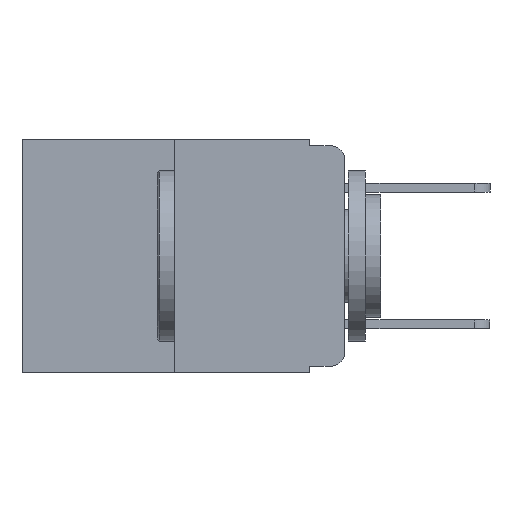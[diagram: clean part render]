
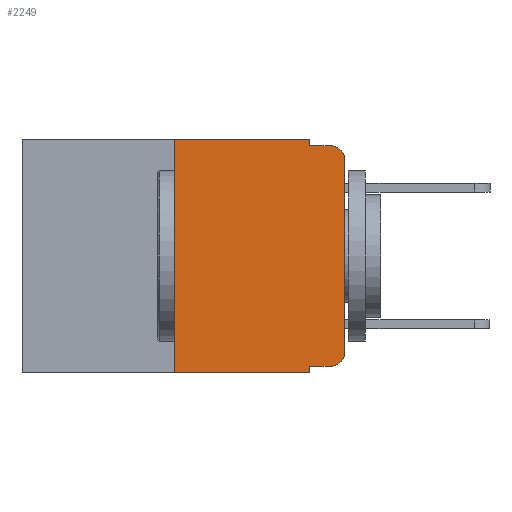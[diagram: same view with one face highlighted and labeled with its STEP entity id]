
A CAD part, left-side view. The second image highlights one B-rep face of the part: STEP entity #2249.
In plain terms, the highlighted planar face has unit normal (-1, 0, 0).
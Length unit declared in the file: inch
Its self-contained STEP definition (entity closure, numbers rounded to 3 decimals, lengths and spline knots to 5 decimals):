
#480 = EDGE_CURVE ( 'NONE', #8708, #18263, #1794, .T. ) ;
#483 = AXIS2_PLACEMENT_3D ( 'NONE', #12032, #5320, #19018 ) ;
#744 = ORIENTED_EDGE ( 'NONE', *, *, #20288, .T. ) ;
#779 = CARTESIAN_POINT ( 'NONE',  ( 0., 0.473, 0. ) ) ;
#816 = ORIENTED_EDGE ( 'NONE', *, *, #19317, .T. ) ;
#1159 = DIRECTION ( 'NONE',  ( 0., -1., 0. ) ) ;
#1303 = ORIENTED_EDGE ( 'NONE', *, *, #17407, .F. ) ;
#1390 = ORIENTED_EDGE ( 'NONE', *, *, #16434, .F. ) ;
#1794 = LINE ( 'NONE', #779, #18004 ) ;
#1799 = ORIENTED_EDGE ( 'NONE', *, *, #480, .F. ) ;
#2011 = LINE ( 'NONE', #6317, #17762 ) ;
#2203 = ORIENTED_EDGE ( 'NONE', *, *, #15414, .F. ) ;
#2249 = ADVANCED_FACE ( 'NONE', ( #18419 ), #9870, .F. ) ;
#2331 = ORIENTED_EDGE ( 'NONE', *, *, #13594, .T. ) ;
#2393 = VERTEX_POINT ( 'NONE', #16743 ) ;
#2771 = DIRECTION ( 'NONE',  ( 0., 0., -1. ) ) ;
#3167 = ORIENTED_EDGE ( 'NONE', *, *, #13340, .F. ) ;
#3249 = CARTESIAN_POINT ( 'NONE',  ( 0., 0.25, 0. ) ) ;
#3755 = ORIENTED_EDGE ( 'NONE', *, *, #12309, .T. ) ;
#3802 = CARTESIAN_POINT ( 'NONE',  ( 0., 0., 0. ) ) ;
#4466 = CARTESIAN_POINT ( 'NONE',  ( 0., 0.051, 0. ) ) ;
#4470 = ORIENTED_EDGE ( 'NONE', *, *, #10319, .T. ) ;
#5081 = VERTEX_POINT ( 'NONE', #13140 ) ;
#5320 = DIRECTION ( 'NONE',  ( 1., 0., 0. ) ) ;
#5491 = DIRECTION ( 'NONE',  ( 0., -1., 0. ) ) ;
#6166 = VECTOR ( 'NONE', #10383, 39.37008 ) ;
#6317 = CARTESIAN_POINT ( 'NONE',  ( 0., 0.051, 0. ) ) ;
#7410 = DIRECTION ( 'NONE',  ( -1., 0., 0. ) ) ;
#7640 = CARTESIAN_POINT ( 'NONE',  ( 0., 0.02, -0.333 ) ) ;
#7674 = EDGE_LOOP ( 'NONE', ( #744, #816, #1303, #1390, #1799, #2203, #2331, #3167, #3755, #4470 ) ) ;
#8078 = LINE ( 'NONE', #12892, #19202 ) ;
#8481 = VECTOR ( 'NONE', #5491, 39.37008 ) ;
#8533 = VERTEX_POINT ( 'NONE', #7640 ) ;
#8648 = VECTOR ( 'NONE', #2771, 39.37008 ) ;
#8708 = VERTEX_POINT ( 'NONE', #9703 ) ;
#9272 = DIRECTION ( 'NONE',  ( -1., 0., 0. ) ) ;
#9484 = CIRCLE ( 'NONE', #16774, 0.02 ) ;
#9703 = CARTESIAN_POINT ( 'NONE',  ( 0., 0.25, 0. ) ) ;
#9870 = PLANE ( 'NONE',  #483 ) ;
#9888 = LINE ( 'NONE', #3249, #13417 ) ;
#10266 = VECTOR ( 'NONE', #17917, 39.37008 ) ;
#10319 = EDGE_CURVE ( 'NONE', #8533, #2393, #19451, .T. ) ;
#10383 = DIRECTION ( 'NONE',  ( 0., 0., 1. ) ) ;
#10418 = LINE ( 'NONE', #3802, #6166 ) ;
#10564 = VERTEX_POINT ( 'NONE', #18702 ) ;
#10792 = CARTESIAN_POINT ( 'NONE',  ( 0., 0.051, 0. ) ) ;
#10928 = CARTESIAN_POINT ( 'NONE',  ( 0., 0.02, -0.01 ) ) ;
#11323 = VERTEX_POINT ( 'NONE', #14184 ) ;
#12032 = CARTESIAN_POINT ( 'NONE',  ( 0., 0.473, 0. ) ) ;
#12309 = EDGE_CURVE ( 'NONE', #5081, #8533, #18733, .T. ) ;
#12691 = LINE ( 'NONE', #4466, #8648 ) ;
#12892 = CARTESIAN_POINT ( 'NONE',  ( 0., 0.051, -0.01 ) ) ;
#13140 = CARTESIAN_POINT ( 'NONE',  ( 0., 0.051, -0.333 ) ) ;
#13340 = EDGE_CURVE ( 'NONE', #5081, #16467, #2011, .T. ) ;
#13417 = VECTOR ( 'NONE', #15945, 39.37008 ) ;
#13594 = EDGE_CURVE ( 'NONE', #15345, #16467, #20012, .T. ) ;
#14184 = CARTESIAN_POINT ( 'NONE',  ( 0., 0.051, -0.01 ) ) ;
#14461 = DIRECTION ( 'NONE',  ( 0., -1., 0. ) ) ;
#14860 = CARTESIAN_POINT ( 'NONE',  ( 0., 0.473, -0.343 ) ) ;
#15126 = AXIS2_PLACEMENT_3D ( 'NONE', #18310, #9272, #19749 ) ;
#15345 = VERTEX_POINT ( 'NONE', #17164 ) ;
#15414 = EDGE_CURVE ( 'NONE', #15345, #8708, #9888, .T. ) ;
#15878 = VERTEX_POINT ( 'NONE', #10928 ) ;
#15945 = DIRECTION ( 'NONE',  ( 0., 0., 1. ) ) ;
#16434 = EDGE_CURVE ( 'NONE', #18263, #11323, #12691, .T. ) ;
#16467 = VERTEX_POINT ( 'NONE', #17064 ) ;
#16487 = CARTESIAN_POINT ( 'NONE',  ( 0., 0.051, -0.333 ) ) ;
#16667 = CARTESIAN_POINT ( 'NONE',  ( 0., 0.02, -0.03 ) ) ;
#16743 = CARTESIAN_POINT ( 'NONE',  ( 0., 0., -0.313 ) ) ;
#16774 = AXIS2_PLACEMENT_3D ( 'NONE', #16667, #7410, #18097 ) ;
#17064 = CARTESIAN_POINT ( 'NONE',  ( 0., 0.051, -0.343 ) ) ;
#17164 = CARTESIAN_POINT ( 'NONE',  ( 0., 0.25, -0.343 ) ) ;
#17407 = EDGE_CURVE ( 'NONE', #11323, #15878, #8078, .T. ) ;
#17762 = VECTOR ( 'NONE', #18584, 39.37008 ) ;
#17917 = DIRECTION ( 'NONE',  ( 0., -1., 0. ) ) ;
#18004 = VECTOR ( 'NONE', #1159, 39.37008 ) ;
#18097 = DIRECTION ( 'NONE',  ( 0., 0., -1. ) ) ;
#18263 = VERTEX_POINT ( 'NONE', #10792 ) ;
#18310 = CARTESIAN_POINT ( 'NONE',  ( 0., 0.02, -0.313 ) ) ;
#18419 = FACE_OUTER_BOUND ( 'NONE', #7674, .T. ) ;
#18584 = DIRECTION ( 'NONE',  ( 0., 0., -1. ) ) ;
#18702 = CARTESIAN_POINT ( 'NONE',  ( 0., 0., -0.03 ) ) ;
#18733 = LINE ( 'NONE', #16487, #10266 ) ;
#19018 = DIRECTION ( 'NONE',  ( 0., 0., -1. ) ) ;
#19202 = VECTOR ( 'NONE', #14461, 39.37008 ) ;
#19317 = EDGE_CURVE ( 'NONE', #10564, #15878, #9484, .T. ) ;
#19451 = CIRCLE ( 'NONE', #15126, 0.02 ) ;
#19749 = DIRECTION ( 'NONE',  ( 0., 0., -1. ) ) ;
#20012 = LINE ( 'NONE', #14860, #8481 ) ;
#20288 = EDGE_CURVE ( 'NONE', #2393, #10564, #10418, .T. ) ;
